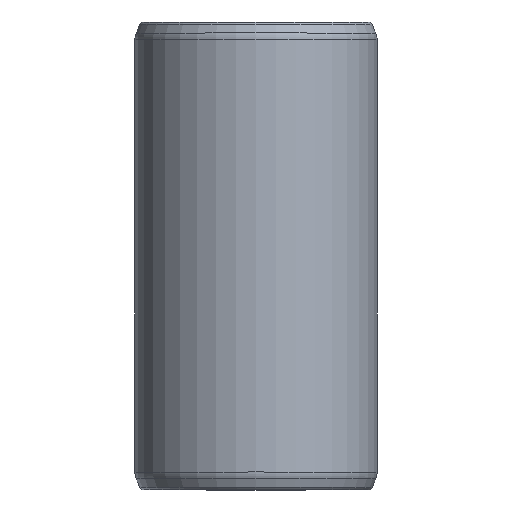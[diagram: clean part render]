
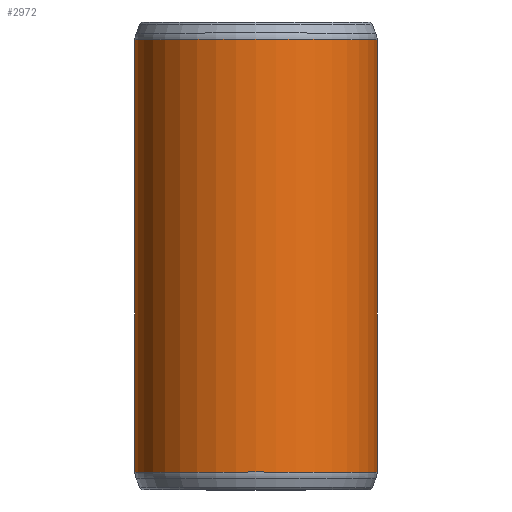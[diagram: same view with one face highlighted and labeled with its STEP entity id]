
A CAD part, top view. The second image highlights one B-rep face of the part: STEP entity #2972.
In plain terms, the highlighted cylindrical face has radius 17.2 mm (diameter 34.4 mm), a partial arc.
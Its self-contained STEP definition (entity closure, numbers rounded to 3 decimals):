
#250=CYLINDRICAL_SURFACE('',#3240,17.2);
#407=FACE_OUTER_BOUND('',#605,.T.);
#605=EDGE_LOOP('',(#2406,#2407,#2408,#2409));
#738=CIRCLE('',#3135,17.2);
#764=CIRCLE('',#3172,17.2);
#875=LINE('',#4537,#1068);
#886=LINE('',#4977,#1079);
#1068=VECTOR('',#3440,10.);
#1079=VECTOR('',#3457,10.);
#1275=VERTEX_POINT('',#4534);
#1276=VERTEX_POINT('',#4536);
#1306=VERTEX_POINT('',#4974);
#1307=VERTEX_POINT('',#4976);
#1553=EDGE_CURVE('',#1275,#1276,#875,.T.);
#1594=EDGE_CURVE('',#1307,#1306,#886,.T.);
#1630=EDGE_CURVE('',#1276,#1306,#738,.T.);
#1667=EDGE_CURVE('',#1307,#1275,#764,.T.);
#2406=ORIENTED_EDGE('',*,*,#1630,.F.);
#2407=ORIENTED_EDGE('',*,*,#1553,.F.);
#2408=ORIENTED_EDGE('',*,*,#1667,.F.);
#2409=ORIENTED_EDGE('',*,*,#1594,.T.);
#2972=ADVANCED_FACE('',(#407),#250,.T.);
#3135=AXIS2_PLACEMENT_3D('',#5365,#3504,#3505);
#3172=AXIS2_PLACEMENT_3D('',#5532,#3582,#3583);
#3240=AXIS2_PLACEMENT_3D('',#5851,#3753,#3754);
#3440=DIRECTION('',(0.,-1.,0.));
#3457=DIRECTION('',(0.,-1.,0.));
#3504=DIRECTION('center_axis',(0.,-1.,0.));
#3505=DIRECTION('ref_axis',(0.,0.,1.));
#3582=DIRECTION('center_axis',(0.,1.,0.));
#3583=DIRECTION('ref_axis',(0.,0.,1.));
#3753=DIRECTION('center_axis',(0.,-1.,0.));
#3754=DIRECTION('ref_axis',(0.,0.,1.));
#4534=CARTESIAN_POINT('',(15.384,160.773,-7.692));
#4536=CARTESIAN_POINT('',(15.384,99.415,-7.692));
#4537=CARTESIAN_POINT('',(15.384,163.45,-7.692));
#4974=CARTESIAN_POINT('',(-15.384,99.415,-7.692));
#4976=CARTESIAN_POINT('',(-15.384,160.773,-7.692));
#4977=CARTESIAN_POINT('',(-15.384,163.45,-7.692));
#5365=CARTESIAN_POINT('Origin',(0.,99.415,0.));
#5532=CARTESIAN_POINT('Origin',(0.,160.773,0.));
#5851=CARTESIAN_POINT('Origin',(0.,163.45,0.));
